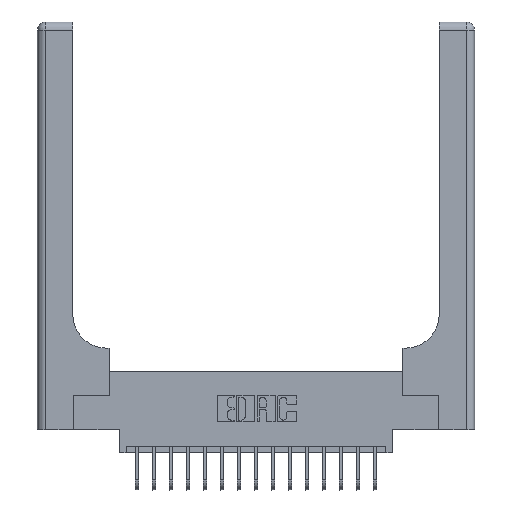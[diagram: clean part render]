
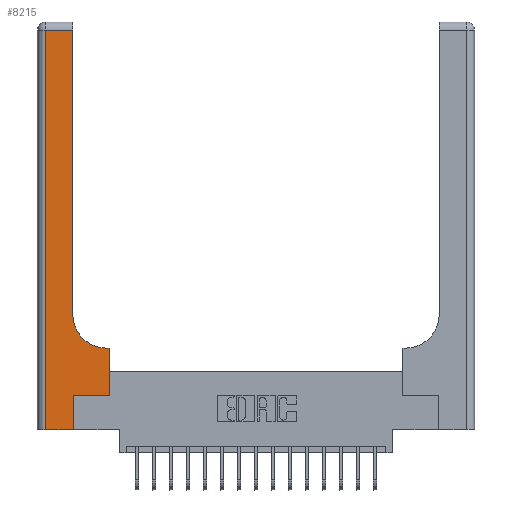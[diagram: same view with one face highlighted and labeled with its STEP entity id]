
A CAD part, top view. The second image highlights one B-rep face of the part: STEP entity #8215.
In plain terms, the highlighted planar face has unit normal (0, 0, 1).
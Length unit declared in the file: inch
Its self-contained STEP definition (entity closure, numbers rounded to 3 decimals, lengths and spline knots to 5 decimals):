
#266 = ORIENTED_EDGE ( 'NONE', *, *, #12845, .T. ) ;
#412 = CARTESIAN_POINT ( 'NONE',  ( 0.06, 2.94, 0.37 ) ) ;
#682 = DIRECTION ( 'NONE',  ( 0., 0., -1. ) ) ;
#763 = EDGE_CURVE ( 'NONE', #8782, #8702, #10857, .T. ) ;
#831 = VECTOR ( 'NONE', #8985, 39.37008 ) ;
#915 = CARTESIAN_POINT ( 'NONE',  ( 0.265, 0., 0.37 ) ) ;
#1080 = EDGE_CURVE ( 'NONE', #16361, #9754, #9724, .T. ) ;
#1140 = ORIENTED_EDGE ( 'NONE', *, *, #12384, .T. ) ;
#1286 = LINE ( 'NONE', #3301, #831 ) ;
#1494 = VERTEX_POINT ( 'NONE', #915 ) ;
#2035 = ORIENTED_EDGE ( 'NONE', *, *, #17460, .T. ) ;
#2384 = CARTESIAN_POINT ( 'NONE',  ( 0.265, 0.25, 0.37 ) ) ;
#2709 = EDGE_CURVE ( 'NONE', #2927, #9532, #1286, .T. ) ;
#2890 = DIRECTION ( 'NONE',  ( 0., 1., 0. ) ) ;
#2899 = CARTESIAN_POINT ( 'NONE',  ( 0., 2.94, 0.37 ) ) ;
#2927 = VERTEX_POINT ( 'NONE', #2384 ) ;
#3233 = VECTOR ( 'NONE', #3282, 39.37008 ) ;
#3256 = CARTESIAN_POINT ( 'NONE',  ( 0.265, 0., 0.37 ) ) ;
#3282 = DIRECTION ( 'NONE',  ( 0., 1., 0. ) ) ;
#3301 = CARTESIAN_POINT ( 'NONE',  ( 0.265, 0.25, 0.37 ) ) ;
#3547 = LINE ( 'NONE', #3256, #6872 ) ;
#3712 = CARTESIAN_POINT ( 'NONE',  ( 0.528, 0.6, 0.37 ) ) ;
#4365 = DIRECTION ( 'NONE',  ( 0., -1., 0. ) ) ;
#4470 = AXIS2_PLACEMENT_3D ( 'NONE', #17670, #682, #10787 ) ;
#4584 = ORIENTED_EDGE ( 'NONE', *, *, #1080, .T. ) ;
#4696 = CARTESIAN_POINT ( 'NONE',  ( 0.528, 0.25, 0.37 ) ) ;
#4835 = ORIENTED_EDGE ( 'NONE', *, *, #763, .T. ) ;
#4864 = DIRECTION ( 'NONE',  ( 0., 0., -1. ) ) ;
#6872 = VECTOR ( 'NONE', #14616, 39.37008 ) ;
#7084 = ORIENTED_EDGE ( 'NONE', *, *, #13100, .T. ) ;
#7216 = FACE_OUTER_BOUND ( 'NONE', #10711, .T. ) ;
#7753 = ORIENTED_EDGE ( 'NONE', *, *, #2709, .T. ) ;
#7866 = PLANE ( 'NONE',  #4470 ) ;
#8215 = ADVANCED_FACE ( 'NONE', ( #7216 ), #7866, .F. ) ;
#8702 = VERTEX_POINT ( 'NONE', #9444 ) ;
#8782 = VERTEX_POINT ( 'NONE', #12664 ) ;
#8985 = DIRECTION ( 'NONE',  ( 1., 0., 0. ) ) ;
#9116 = CARTESIAN_POINT ( 'NONE',  ( 0.26, 0.6, 0.37 ) ) ;
#9260 = VECTOR ( 'NONE', #4365, 39.37008 ) ;
#9444 = CARTESIAN_POINT ( 'NONE',  ( 0.26, 0.85, 0.37 ) ) ;
#9532 = VERTEX_POINT ( 'NONE', #15632 ) ;
#9724 = LINE ( 'NONE', #15659, #9260 ) ;
#9754 = VERTEX_POINT ( 'NONE', #12012 ) ;
#9870 = CARTESIAN_POINT ( 'NONE',  ( 0., 0., 0.37 ) ) ;
#10111 = CARTESIAN_POINT ( 'NONE',  ( 0.26, 3., 0.37 ) ) ;
#10191 = LINE ( 'NONE', #9870, #13927 ) ;
#10711 = EDGE_LOOP ( 'NONE', ( #2035, #16871, #4584, #266, #1140, #7753, #7084, #16150, #4835 ) ) ;
#10787 = DIRECTION ( 'NONE',  ( -1., 0., 0. ) ) ;
#10855 = LINE ( 'NONE', #4696, #3233 ) ;
#10857 = CIRCLE ( 'NONE', #16381, 0.25 ) ;
#11594 = LINE ( 'NONE', #10111, #14440 ) ;
#11888 = VECTOR ( 'NONE', #11974, 39.37008 ) ;
#11974 = DIRECTION ( 'NONE',  ( -1., 0., 0. ) ) ;
#12012 = CARTESIAN_POINT ( 'NONE',  ( 0.06, 0., 0.37 ) ) ;
#12093 = VERTEX_POINT ( 'NONE', #13593 ) ;
#12112 = VERTEX_POINT ( 'NONE', #3712 ) ;
#12155 = VECTOR ( 'NONE', #15689, 39.37008 ) ;
#12384 = EDGE_CURVE ( 'NONE', #1494, #2927, #3547, .T. ) ;
#12664 = CARTESIAN_POINT ( 'NONE',  ( 0.51, 0.6, 0.37 ) ) ;
#12845 = EDGE_CURVE ( 'NONE', #9754, #1494, #10191, .T. ) ;
#12971 = EDGE_CURVE ( 'NONE', #12093, #16361, #15880, .T. ) ;
#13100 = EDGE_CURVE ( 'NONE', #9532, #12112, #10855, .T. ) ;
#13401 = CARTESIAN_POINT ( 'NONE',  ( 0.51, 0.85, 0.37 ) ) ;
#13593 = CARTESIAN_POINT ( 'NONE',  ( 0.26, 2.94, 0.37 ) ) ;
#13927 = VECTOR ( 'NONE', #18186, 39.37008 ) ;
#14267 = EDGE_CURVE ( 'NONE', #12112, #8782, #15612, .T. ) ;
#14440 = VECTOR ( 'NONE', #2890, 39.37008 ) ;
#14616 = DIRECTION ( 'NONE',  ( 0., 1., 0. ) ) ;
#14815 = DIRECTION ( 'NONE',  ( 1., 0., 0. ) ) ;
#15612 = LINE ( 'NONE', #9116, #11888 ) ;
#15632 = CARTESIAN_POINT ( 'NONE',  ( 0.528, 0.25, 0.37 ) ) ;
#15659 = CARTESIAN_POINT ( 'NONE',  ( 0.06, 3., 0.37 ) ) ;
#15689 = DIRECTION ( 'NONE',  ( -1., 0., 0. ) ) ;
#15880 = LINE ( 'NONE', #2899, #12155 ) ;
#16150 = ORIENTED_EDGE ( 'NONE', *, *, #14267, .T. ) ;
#16361 = VERTEX_POINT ( 'NONE', #412 ) ;
#16381 = AXIS2_PLACEMENT_3D ( 'NONE', #13401, #4864, #14815 ) ;
#16871 = ORIENTED_EDGE ( 'NONE', *, *, #12971, .T. ) ;
#17460 = EDGE_CURVE ( 'NONE', #8702, #12093, #11594, .T. ) ;
#17670 = CARTESIAN_POINT ( 'NONE',  ( 0., 3., 0.37 ) ) ;
#18186 = DIRECTION ( 'NONE',  ( 1., 0., 0. ) ) ;
